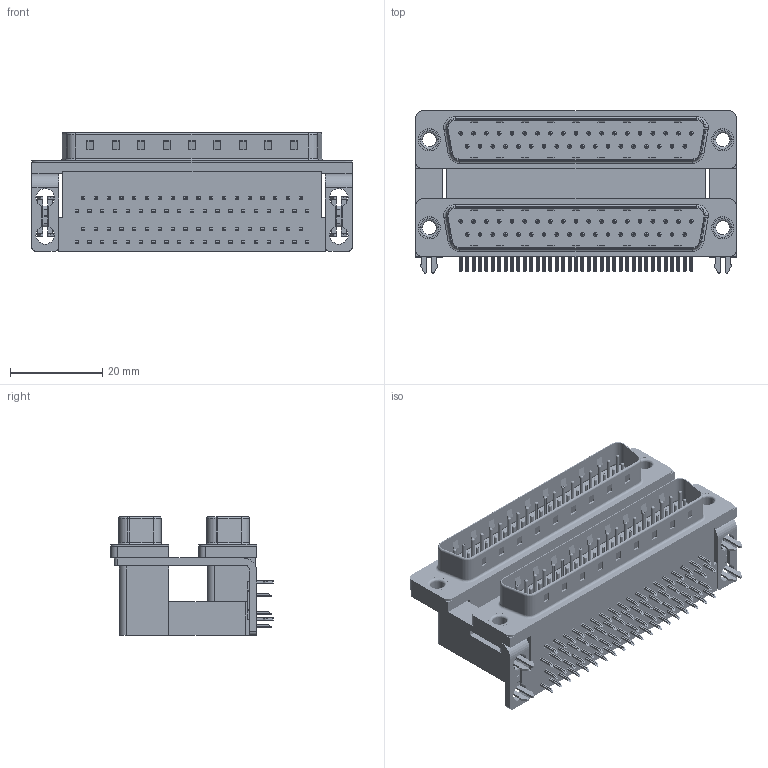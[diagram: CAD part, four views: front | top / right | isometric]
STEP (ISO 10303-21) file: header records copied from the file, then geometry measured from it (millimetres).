
FILE_DESCRIPTION (( 'STEP AP203' ), '1' );
FILE_NAME ('661-037-364-037.STEP', '2022-06-15T21:53:59', ( '' ), ( '' ), 'SwSTEP 2.0', 'SolidWorks 2020', '' );
FILE_SCHEMA (( 'CONFIG_CONTROL_DESIGN' ));
Length unit declared in the file: millimetre
Products named in the file (12): 661 Mounting Bracket_2ProngM; 661 Shell_37 Contacts; 661-037-364-037; 661 Thru Hole Rivet; 661 2 Prong Board Lock_3; 661 Contact Top Lower; 661 Contact Bottom Upper_M; 661 Housing Spacer_37 Contacts M; 661 Contact Bottom Lower; 661 Housing Upper_37 Contacts M; 661 Housing Lower_37 Contacts; 661 Contact Top Upper_M
Assembly tree (87 placements, depth 2):
  661-037-364-037
    661 Housing Lower_37 Contacts
    661 Housing Spacer_37 Contacts M
    661 Housing Upper_37 Contacts M
    661 Shell_37 Contacts  x2
    661 Contact Bottom Lower  x18
    661 Contact Top Lower  x19
    661 Contact Bottom Upper_M  x18
    661 Contact Top Upper_M  x19
    661 Mounting Bracket_2ProngM  x2
    661 2 Prong Board Lock_3  x2
    661 Thru Hole Rivet  x4
Bounding box: 69.32 x 35.1 x 25.6 mm (x, y, z)
Volume: 29231 mm3; surface area: 29957 mm2
Topology: 87 solids, 87 shells, 6650 faces, 16542 edges, 10238 vertices
Faces by surface type: plane 4352, cylinder 1808, torus 490
Entity records: 50967 total; most frequent: CARTESIAN_POINT 8286, DIRECTION 8105, ORIENTED_EDGE 7966, EDGE_CURVE 3983, VECTOR 3157, LINE 3157, VERTEX_POINT 2591, AXIS2_PLACEMENT_3D 2474
